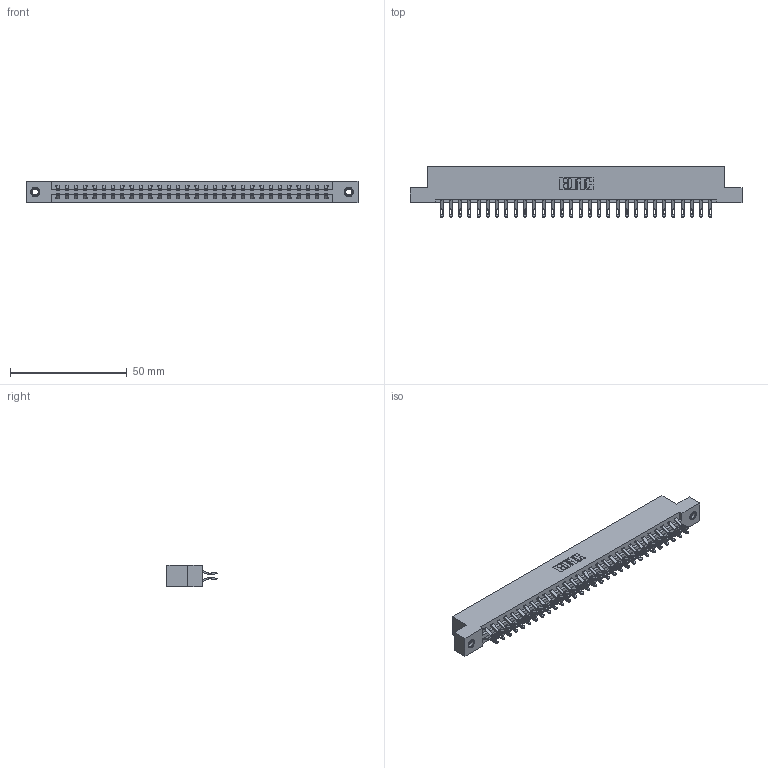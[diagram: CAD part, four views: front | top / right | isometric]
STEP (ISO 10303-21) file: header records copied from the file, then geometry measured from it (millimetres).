
FILE_DESCRIPTION (( 'STEP AP203' ), '1' );
FILE_NAME ('387-060-555-207.STEP', '2019-10-19T13:56:37', ( '' ), ( '' ), 'SwSTEP 2.0', 'SolidWorks 2016', '' );
FILE_SCHEMA (( 'CONFIG_CONTROL_DESIGN' ));
Length unit declared in the file: inch
Products named in the file (4): 337 Part_Flush Mounting Lugs - 0.156 Dia-TI; 345-292-001_555 Tail; 345-250-001_345-250-005-103; 387-060-555-207
Assembly tree (63 placements, depth 2):
  387-060-555-207
    337 Part_Flush Mounting Lugs - 0.156 Dia-TI
    345-292-001_555 Tail  x60
    345-250-001_345-250-005-103  x2
Bounding box: 141.88 x 21.47 x 9.4 mm (x, y, z)
Volume: 14953.7 mm3; surface area: 17480.4 mm2
Topology: 63 solids, 63 shells, 3774 faces, 11787 edges, 7850 vertices
Faces by surface type: plane 2262, cylinder 1496, cone 12, torus 4
Entity records: 26324 total; most frequent: CARTESIAN_POINT 4459, ORIENTED_EDGE 4358, DIRECTION 3817, EDGE_CURVE 2179, VECTOR 2011, LINE 2011, VERTEX_POINT 1448, AXIS2_PLACEMENT_3D 903
